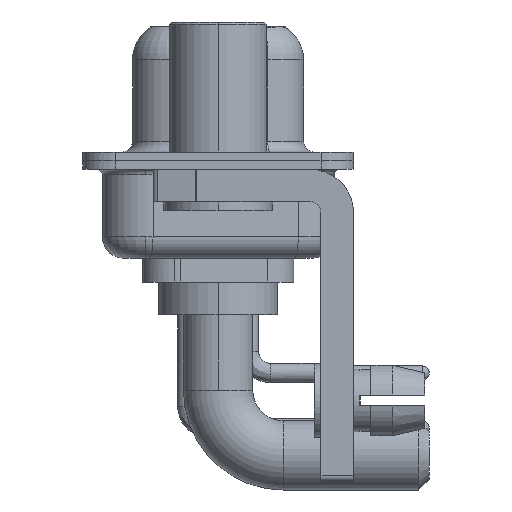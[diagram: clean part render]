
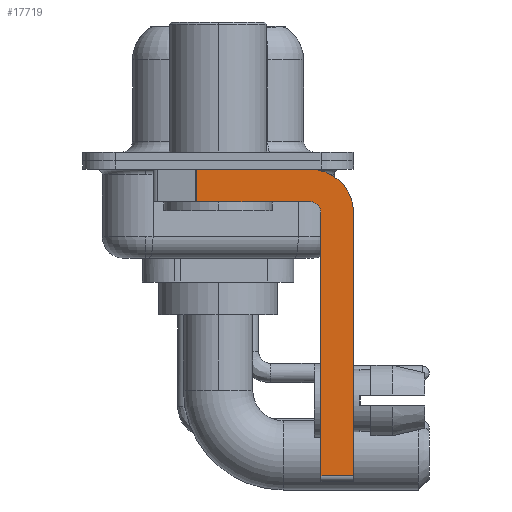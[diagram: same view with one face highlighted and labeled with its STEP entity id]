
A CAD part, left-side view. The second image highlights one B-rep face of the part: STEP entity #17719.
In plain terms, the highlighted planar face has unit normal (-1, 0, 0).
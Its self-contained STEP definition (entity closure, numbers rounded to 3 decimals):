
#14 = ORIENTED_EDGE ( 'NONE', *, *, #10147, .T. ) ;
#461 = DIRECTION ( 'NONE',  ( 1., 0., 0. ) ) ;
#666 = CARTESIAN_POINT ( 'NONE',  ( -2.9, -4.25, -0.4 ) ) ;
#950 = VECTOR ( 'NONE', #5978, 1000. ) ;
#996 = LINE ( 'NONE', #9927, #7697 ) ;
#1135 = LINE ( 'NONE', #2904, #8803 ) ;
#1869 = DIRECTION ( 'NONE',  ( 1., 0., 0. ) ) ;
#2001 = EDGE_CURVE ( 'NONE', #4132, #22586, #12398, .T. ) ;
#2422 = EDGE_CURVE ( 'NONE', #3612, #4132, #14331, .T. ) ;
#2904 = CARTESIAN_POINT ( 'NONE',  ( -2.9, 3., -0.4 ) ) ;
#3441 = DIRECTION ( 'NONE',  ( 0., 0., 1. ) ) ;
#3612 = VERTEX_POINT ( 'NONE', #19710 ) ;
#3638 = LINE ( 'NONE', #10571, #14839 ) ;
#3647 = FACE_OUTER_BOUND ( 'NONE', #7598, .T. ) ;
#4132 = VERTEX_POINT ( 'NONE', #5953 ) ;
#4854 = DIRECTION ( 'NONE',  ( -1., 0., 0. ) ) ;
#5340 = AXIS2_PLACEMENT_3D ( 'NONE', #21473, #1869, #14425 ) ;
#5747 = LINE ( 'NONE', #11131, #950 ) ;
#5953 = CARTESIAN_POINT ( 'NONE',  ( -2.9, -4.75, -2.4 ) ) ;
#5978 = DIRECTION ( 'NONE',  ( 0., 1., 0. ) ) ;
#6445 = VECTOR ( 'NONE', #3441, 1000. ) ;
#6784 = DIRECTION ( 'NONE',  ( 0., -1., 0. ) ) ;
#6887 = ORIENTED_EDGE ( 'NONE', *, *, #12627, .F. ) ;
#7392 = PLANE ( 'NONE',  #5340 ) ;
#7501 = CIRCLE ( 'NONE', #20614, 2. ) ;
#7516 = CARTESIAN_POINT ( 'NONE',  ( -2.9, -6.25, -2.4 ) ) ;
#7598 = EDGE_LOOP ( 'NONE', ( #13017, #9872, #15232, #21967, #20472, #14, #15543, #6887 ) ) ;
#7697 = VECTOR ( 'NONE', #8173, 1000. ) ;
#8173 = DIRECTION ( 'NONE',  ( 0., 0., -1. ) ) ;
#8310 = VERTEX_POINT ( 'NONE', #666 ) ;
#8382 = EDGE_CURVE ( 'NONE', #17759, #8310, #1135, .T. ) ;
#8474 = LINE ( 'NONE', #13502, #17803 ) ;
#8616 = DIRECTION ( 'NONE',  ( 0., 0., 1. ) ) ;
#8803 = VECTOR ( 'NONE', #6784, 1000. ) ;
#9298 = CARTESIAN_POINT ( 'NONE',  ( -2.9, -4.75, -14.8 ) ) ;
#9617 = EDGE_CURVE ( 'NONE', #12717, #13434, #996, .T. ) ;
#9872 = ORIENTED_EDGE ( 'NONE', *, *, #22238, .T. ) ;
#9927 = CARTESIAN_POINT ( 'NONE',  ( -2.9, -6.25, -2.4 ) ) ;
#10147 = EDGE_CURVE ( 'NONE', #3612, #13434, #3638, .T. ) ;
#10571 = CARTESIAN_POINT ( 'NONE',  ( -2.9, -4.25, -14.55 ) ) ;
#10808 = CARTESIAN_POINT ( 'NONE',  ( -2.9, -4.25, -2.4 ) ) ;
#11131 = CARTESIAN_POINT ( 'NONE',  ( -2.9, -4.25, -1.9 ) ) ;
#11693 = VERTEX_POINT ( 'NONE', #20355 ) ;
#12398 = CIRCLE ( 'NONE', #22901, 0.5 ) ;
#12447 = DIRECTION ( 'NONE',  ( 0., -1., 0. ) ) ;
#12627 = EDGE_CURVE ( 'NONE', #8310, #12717, #7501, .T. ) ;
#12717 = VERTEX_POINT ( 'NONE', #7516 ) ;
#12893 = CARTESIAN_POINT ( 'NONE',  ( -2.9, -4.25, -1.9 ) ) ;
#13017 = ORIENTED_EDGE ( 'NONE', *, *, #8382, .F. ) ;
#13434 = VERTEX_POINT ( 'NONE', #19554 ) ;
#13502 = CARTESIAN_POINT ( 'NONE',  ( -2.9, 0.978, -1.9 ) ) ;
#14331 = LINE ( 'NONE', #9298, #6445 ) ;
#14425 = DIRECTION ( 'NONE',  ( 0., 0., -1. ) ) ;
#14839 = VECTOR ( 'NONE', #12447, 1000. ) ;
#15232 = ORIENTED_EDGE ( 'NONE', *, *, #22540, .F. ) ;
#15543 = ORIENTED_EDGE ( 'NONE', *, *, #9617, .F. ) ;
#17719 = ADVANCED_FACE ( 'NONE', ( #3647 ), #7392, .F. ) ;
#17759 = VERTEX_POINT ( 'NONE', #17950 ) ;
#17803 = VECTOR ( 'NONE', #19242, 1000. ) ;
#17950 = CARTESIAN_POINT ( 'NONE',  ( -2.9, 0.978, -0.4 ) ) ;
#19242 = DIRECTION ( 'NONE',  ( 0., 0., -1. ) ) ;
#19554 = CARTESIAN_POINT ( 'NONE',  ( -2.9, -6.25, -14.55 ) ) ;
#19710 = CARTESIAN_POINT ( 'NONE',  ( -2.9, -4.75, -14.55 ) ) ;
#20060 = DIRECTION ( 'NONE',  ( 0., 0., -1. ) ) ;
#20355 = CARTESIAN_POINT ( 'NONE',  ( -2.9, 0.978, -1.9 ) ) ;
#20472 = ORIENTED_EDGE ( 'NONE', *, *, #2422, .F. ) ;
#20614 = AXIS2_PLACEMENT_3D ( 'NONE', #10808, #461, #20060 ) ;
#20807 = CARTESIAN_POINT ( 'NONE',  ( -2.9, -4.25, -2.4 ) ) ;
#21473 = CARTESIAN_POINT ( 'NONE',  ( -2.9, -4.25, -2.4 ) ) ;
#21967 = ORIENTED_EDGE ( 'NONE', *, *, #2001, .F. ) ;
#22238 = EDGE_CURVE ( 'NONE', #17759, #11693, #8474, .T. ) ;
#22540 = EDGE_CURVE ( 'NONE', #22586, #11693, #5747, .T. ) ;
#22586 = VERTEX_POINT ( 'NONE', #12893 ) ;
#22901 = AXIS2_PLACEMENT_3D ( 'NONE', #20807, #4854, #8616 ) ;
